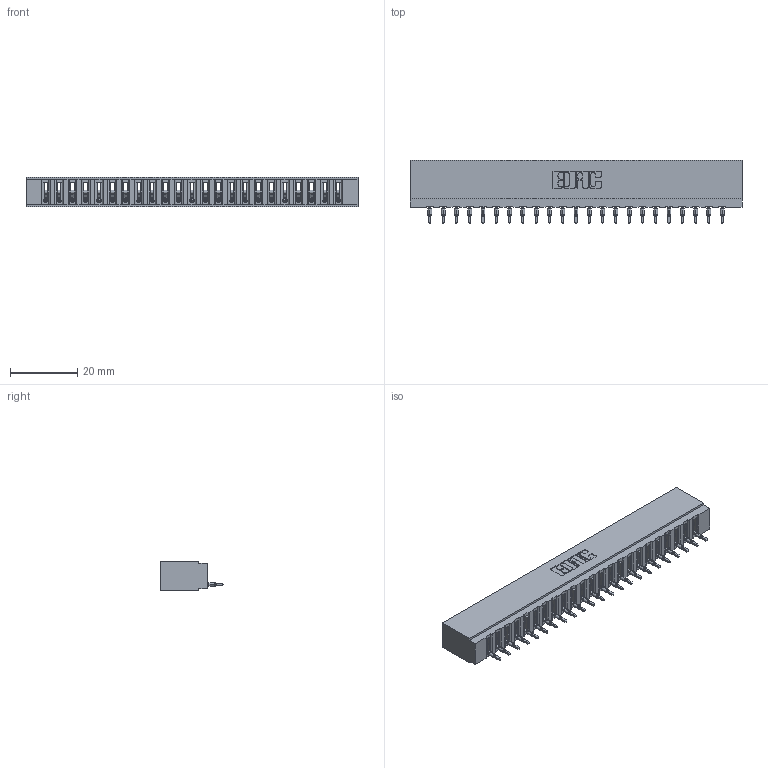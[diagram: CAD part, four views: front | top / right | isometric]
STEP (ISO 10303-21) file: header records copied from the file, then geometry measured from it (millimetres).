
FILE_DESCRIPTION (( 'STEP AP203' ), '1' );
FILE_NAME ('717-023-560-106.STEP', '2020-03-13T19:31:57', ( '' ), ( '' ), 'SwSTEP 2.0', 'SolidWorks 2016', '' );
FILE_SCHEMA (( 'CONFIG_CONTROL_DESIGN' ));
Length unit declared in the file: inch
Products named in the file (3): 745-292-001_560; 717 Part_Insulator Option - 06; 717-023-560-106
Assembly tree (24 placements, depth 2):
  717-023-560-106
    717 Part_Insulator Option - 06
    745-292-001_560  x23
Bounding box: 99.01 x 18.78 x 8.89 mm (x, y, z)
Volume: 8517.3 mm3; surface area: 12130.6 mm2
Topology: 24 solids, 24 shells, 2900 faces, 8071 edges, 5134 vertices
Faces by surface type: plane 1733, cylinder 569, bspline 460, torus 138
Entity records: 41598 total; most frequent: CARTESIAN_POINT 7834, ORIENTED_EDGE 7254, DIRECTION 6309, EDGE_CURVE 3627, LINE 3299, VECTOR 3299, VERTEX_POINT 2318, AXIS2_PLACEMENT_3D 1505
